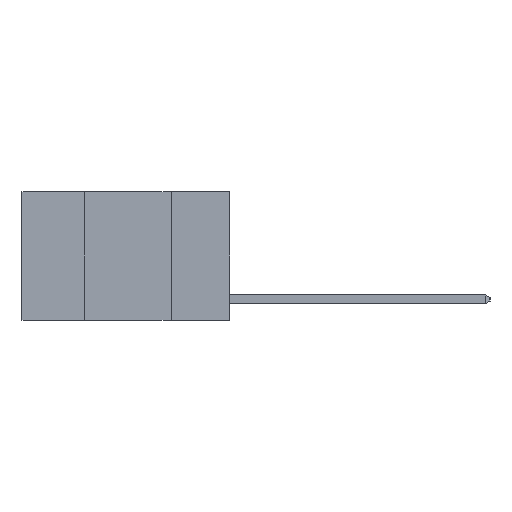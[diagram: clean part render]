
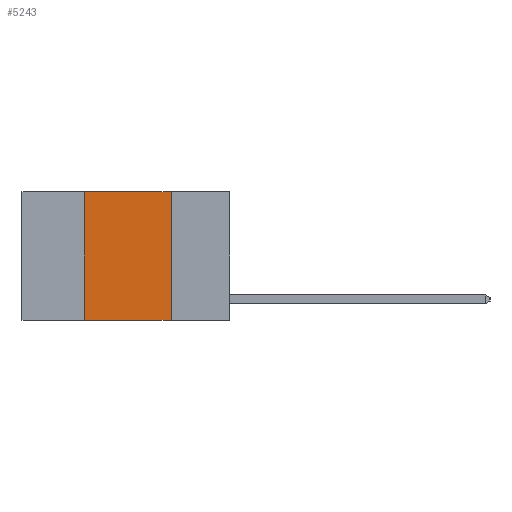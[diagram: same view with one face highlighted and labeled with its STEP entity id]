
A CAD part, left-side view. The second image highlights one B-rep face of the part: STEP entity #5243.
In plain terms, the highlighted planar face has unit normal (-1, 0, 0).
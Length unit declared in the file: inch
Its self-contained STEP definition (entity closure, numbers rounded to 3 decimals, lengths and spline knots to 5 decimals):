
#6 = CARTESIAN_POINT ( 'NONE',  ( 0., 0.42, 0. ) ) ;
#41 = ORIENTED_EDGE ( 'NONE', *, *, #650, .F. ) ;
#92 = CARTESIAN_POINT ( 'NONE',  ( 0., 0.17, -0.37 ) ) ;
#179 = VERTEX_POINT ( 'NONE', #92 ) ;
#199 = ORIENTED_EDGE ( 'NONE', *, *, #11600, .F. ) ;
#650 = EDGE_CURVE ( 'NONE', #6605, #179, #2313, .T. ) ;
#912 = FACE_OUTER_BOUND ( 'NONE', #11155, .T. ) ;
#1733 = EDGE_CURVE ( 'NONE', #2347, #179, #10024, .T. ) ;
#1840 = PLANE ( 'NONE',  #11380 ) ;
#2071 = VECTOR ( 'NONE', #9491, 39.37008 ) ;
#2122 = EDGE_CURVE ( 'NONE', #2347, #9013, #8166, .T. ) ;
#2313 = LINE ( 'NONE', #5354, #11744 ) ;
#2340 = DIRECTION ( 'NONE',  ( 0., -1., 0. ) ) ;
#2347 = VERTEX_POINT ( 'NONE', #4198 ) ;
#2718 = VECTOR ( 'NONE', #2340, 39.37008 ) ;
#3085 = CARTESIAN_POINT ( 'NONE',  ( 0., 0.6, 0. ) ) ;
#3109 = ORIENTED_EDGE ( 'NONE', *, *, #2122, .F. ) ;
#3717 = DIRECTION ( 'NONE',  ( 0., 0., 1. ) ) ;
#4198 = CARTESIAN_POINT ( 'NONE',  ( 0., 0.42, -0.37 ) ) ;
#4346 = CARTESIAN_POINT ( 'NONE',  ( 0., 0.42, 0. ) ) ;
#4636 = DIRECTION ( 'NONE',  ( 1., 0., 0. ) ) ;
#5243 = ADVANCED_FACE ( 'NONE', ( #912 ), #1840, .F. ) ;
#5354 = CARTESIAN_POINT ( 'NONE',  ( 0., 0.17, 0. ) ) ;
#5695 = VECTOR ( 'NONE', #3717, 39.37008 ) ;
#6605 = VERTEX_POINT ( 'NONE', #10712 ) ;
#6737 = ORIENTED_EDGE ( 'NONE', *, *, #1733, .T. ) ;
#7837 = CARTESIAN_POINT ( 'NONE',  ( 0., 0.6, -0.37 ) ) ;
#8166 = LINE ( 'NONE', #6, #5695 ) ;
#9013 = VERTEX_POINT ( 'NONE', #4346 ) ;
#9055 = DIRECTION ( 'NONE',  ( 0., 0., -1. ) ) ;
#9099 = LINE ( 'NONE', #3085, #2071 ) ;
#9491 = DIRECTION ( 'NONE',  ( 0., -1., 0. ) ) ;
#10024 = LINE ( 'NONE', #7837, #2718 ) ;
#10114 = CARTESIAN_POINT ( 'NONE',  ( 0., 0.6, 0. ) ) ;
#10712 = CARTESIAN_POINT ( 'NONE',  ( 0., 0.17, 0. ) ) ;
#11029 = DIRECTION ( 'NONE',  ( 0., 0., -1. ) ) ;
#11155 = EDGE_LOOP ( 'NONE', ( #41, #199, #3109, #6737 ) ) ;
#11380 = AXIS2_PLACEMENT_3D ( 'NONE', #10114, #4636, #11029 ) ;
#11600 = EDGE_CURVE ( 'NONE', #9013, #6605, #9099, .T. ) ;
#11744 = VECTOR ( 'NONE', #9055, 39.37008 ) ;
